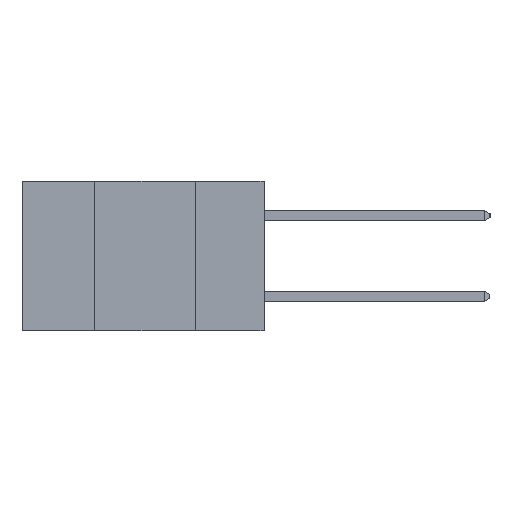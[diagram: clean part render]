
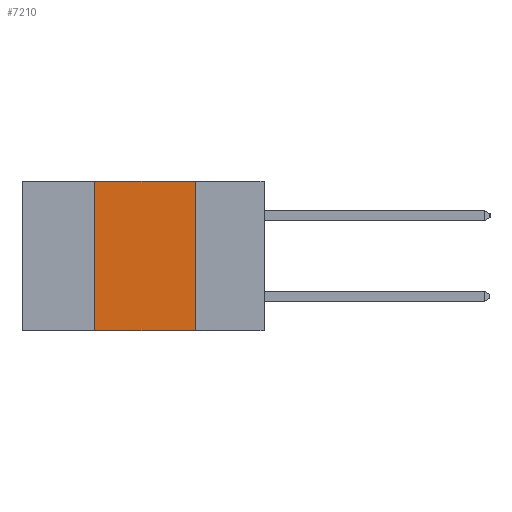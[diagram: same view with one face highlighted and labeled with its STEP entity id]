
A CAD part, left-side view. The second image highlights one B-rep face of the part: STEP entity #7210.
In plain terms, the highlighted planar face has unit normal (-1, 0, 0).
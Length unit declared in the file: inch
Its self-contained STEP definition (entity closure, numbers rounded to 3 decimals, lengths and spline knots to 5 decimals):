
#214 = ORIENTED_EDGE ( 'NONE', *, *, #1470, .T. ) ;
#331 = VERTEX_POINT ( 'NONE', #8058 ) ;
#1235 = DIRECTION ( 'NONE',  ( 0., 0., 1. ) ) ;
#1330 = VERTEX_POINT ( 'NONE', #7388 ) ;
#1470 = EDGE_CURVE ( 'NONE', #331, #1330, #7576, .T. ) ;
#1517 = EDGE_CURVE ( 'NONE', #16101, #5347, #2577, .T. ) ;
#1612 = FACE_OUTER_BOUND ( 'NONE', #11392, .T. ) ;
#2289 = DIRECTION ( 'NONE',  ( 0., -1., 0. ) ) ;
#2394 = VECTOR ( 'NONE', #7956, 39.37008 ) ;
#2577 = LINE ( 'NONE', #16620, #8727 ) ;
#3129 = DIRECTION ( 'NONE',  ( 1., 0., 0. ) ) ;
#3572 = DIRECTION ( 'NONE',  ( 0., 0., -1. ) ) ;
#4382 = VECTOR ( 'NONE', #1235, 39.37008 ) ;
#4448 = DIRECTION ( 'NONE',  ( 0., 0., -1. ) ) ;
#4556 = ORIENTED_EDGE ( 'NONE', *, *, #5935, .F. ) ;
#4889 = CARTESIAN_POINT ( 'NONE',  ( 0., 0.42, 0. ) ) ;
#5347 = VERTEX_POINT ( 'NONE', #17628 ) ;
#5935 = EDGE_CURVE ( 'NONE', #5347, #1330, #7721, .T. ) ;
#7210 = ADVANCED_FACE ( 'NONE', ( #1612 ), #11630, .F. ) ;
#7388 = CARTESIAN_POINT ( 'NONE',  ( 0., 0.17, -0.37 ) ) ;
#7576 = LINE ( 'NONE', #7772, #2394 ) ;
#7721 = LINE ( 'NONE', #7910, #12707 ) ;
#7772 = CARTESIAN_POINT ( 'NONE',  ( 0., 0.6, -0.37 ) ) ;
#7910 = CARTESIAN_POINT ( 'NONE',  ( 0., 0.17, -0.37 ) ) ;
#7956 = DIRECTION ( 'NONE',  ( 0., -1., 0. ) ) ;
#8058 = CARTESIAN_POINT ( 'NONE',  ( 0., 0.42, -0.37 ) ) ;
#8727 = VECTOR ( 'NONE', #2289, 39.37008 ) ;
#11392 = EDGE_LOOP ( 'NONE', ( #4556, #16775, #15448, #214 ) ) ;
#11630 = PLANE ( 'NONE',  #13927 ) ;
#12707 = VECTOR ( 'NONE', #3572, 39.37008 ) ;
#13927 = AXIS2_PLACEMENT_3D ( 'NONE', #14253, #3129, #4448 ) ;
#14139 = CARTESIAN_POINT ( 'NONE',  ( 0., 0.42, -0.37 ) ) ;
#14253 = CARTESIAN_POINT ( 'NONE',  ( 0., 0.6, 0. ) ) ;
#15448 = ORIENTED_EDGE ( 'NONE', *, *, #15809, .F. ) ;
#15809 = EDGE_CURVE ( 'NONE', #331, #16101, #18103, .T. ) ;
#16101 = VERTEX_POINT ( 'NONE', #4889 ) ;
#16620 = CARTESIAN_POINT ( 'NONE',  ( 0., 0.6, 0. ) ) ;
#16775 = ORIENTED_EDGE ( 'NONE', *, *, #1517, .F. ) ;
#17628 = CARTESIAN_POINT ( 'NONE',  ( 0., 0.17, 0. ) ) ;
#18103 = LINE ( 'NONE', #14139, #4382 ) ;
